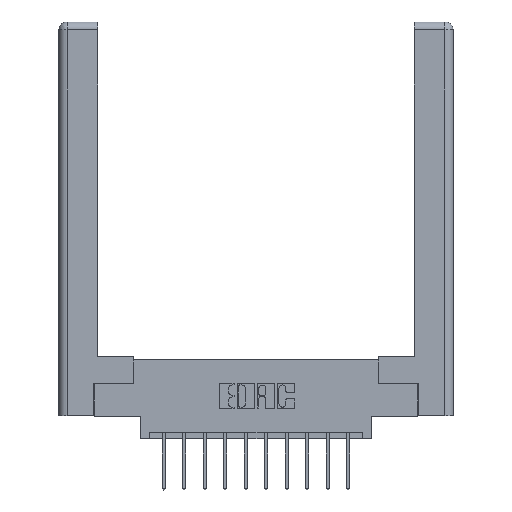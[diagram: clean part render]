
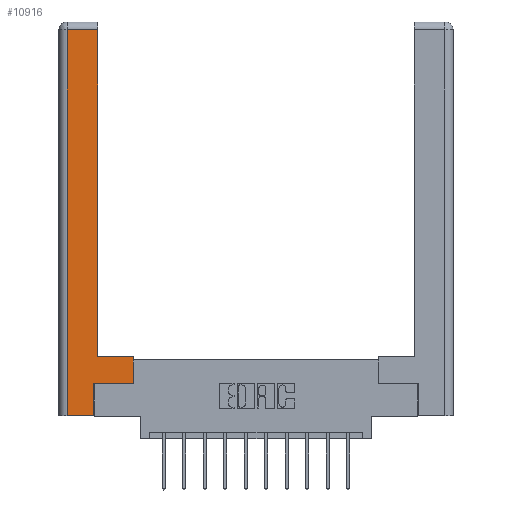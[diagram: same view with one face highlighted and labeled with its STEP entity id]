
A CAD part, top view. The second image highlights one B-rep face of the part: STEP entity #10916.
In plain terms, the highlighted planar face has unit normal (0, 0, 1).
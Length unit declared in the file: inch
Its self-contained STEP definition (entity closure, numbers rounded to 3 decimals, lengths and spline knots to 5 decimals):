
#333 = VECTOR ( 'NONE', #755, 39.37008 ) ;
#377 = LINE ( 'NONE', #9315, #12081 ) ;
#511 = VERTEX_POINT ( 'NONE', #4430 ) ;
#755 = DIRECTION ( 'NONE',  ( 0., -1., 0. ) ) ;
#834 = DIRECTION ( 'NONE',  ( -1., 0., 0. ) ) ;
#1196 = LINE ( 'NONE', #2316, #3840 ) ;
#1319 = VERTEX_POINT ( 'NONE', #8373 ) ;
#1495 = DIRECTION ( 'NONE',  ( -1., 0., 0. ) ) ;
#1690 = LINE ( 'NONE', #4418, #2929 ) ;
#2316 = CARTESIAN_POINT ( 'NONE',  ( 0.265, 0., 0. ) ) ;
#2762 = ORIENTED_EDGE ( 'NONE', *, *, #9810, .T. ) ;
#2822 = EDGE_CURVE ( 'NONE', #14529, #1319, #4258, .T. ) ;
#2929 = VECTOR ( 'NONE', #7453, 39.37008 ) ;
#3008 = FACE_OUTER_BOUND ( 'NONE', #6752, .T. ) ;
#3546 = EDGE_CURVE ( 'NONE', #511, #11935, #4234, .T. ) ;
#3840 = VECTOR ( 'NONE', #12680, 39.37008 ) ;
#3909 = PLANE ( 'NONE',  #6872 ) ;
#4000 = CARTESIAN_POINT ( 'NONE',  ( 0.295, 2.94, 0. ) ) ;
#4083 = CARTESIAN_POINT ( 'NONE',  ( 0.0615, 0., 0. ) ) ;
#4232 = ORIENTED_EDGE ( 'NONE', *, *, #2822, .T. ) ;
#4234 = LINE ( 'NONE', #9967, #333 ) ;
#4258 = LINE ( 'NONE', #5767, #7293 ) ;
#4418 = CARTESIAN_POINT ( 'NONE',  ( 0.265, 0.245, 0. ) ) ;
#4430 = CARTESIAN_POINT ( 'NONE',  ( 0.0615, 2.94, 0. ) ) ;
#4433 = CARTESIAN_POINT ( 'NONE',  ( 0.295, 0.45, 0. ) ) ;
#4456 = LINE ( 'NONE', #5331, #5339 ) ;
#4597 = CARTESIAN_POINT ( 'NONE',  ( 0.565, 0.45, 0. ) ) ;
#4698 = DIRECTION ( 'NONE',  ( 0., 1., 0. ) ) ;
#5149 = LINE ( 'NONE', #12906, #12946 ) ;
#5331 = CARTESIAN_POINT ( 'NONE',  ( 0.0615, 2.94, 0. ) ) ;
#5339 = VECTOR ( 'NONE', #834, 39.37008 ) ;
#5767 = CARTESIAN_POINT ( 'NONE',  ( 0.565, 0.245, 0. ) ) ;
#6020 = DIRECTION ( 'NONE',  ( -1., 0., 0. ) ) ;
#6538 = ORIENTED_EDGE ( 'NONE', *, *, #12284, .T. ) ;
#6570 = ORIENTED_EDGE ( 'NONE', *, *, #8959, .T. ) ;
#6721 = VERTEX_POINT ( 'NONE', #4597 ) ;
#6752 = EDGE_LOOP ( 'NONE', ( #6570, #8140, #14511, #6538, #13121, #4232, #2762, #13319 ) ) ;
#6872 = AXIS2_PLACEMENT_3D ( 'NONE', #14090, #10619, #1495 ) ;
#7293 = VECTOR ( 'NONE', #12496, 39.37008 ) ;
#7317 = DIRECTION ( 'NONE',  ( 0., 1., 0. ) ) ;
#7453 = DIRECTION ( 'NONE',  ( 0., 1., 0. ) ) ;
#8140 = ORIENTED_EDGE ( 'NONE', *, *, #9294, .T. ) ;
#8185 = VERTEX_POINT ( 'NONE', #4000 ) ;
#8361 = CARTESIAN_POINT ( 'NONE',  ( 0.295, 0.45, 0. ) ) ;
#8373 = CARTESIAN_POINT ( 'NONE',  ( 0.565, 0.245, 0. ) ) ;
#8959 = EDGE_CURVE ( 'NONE', #11451, #8185, #377, .T. ) ;
#9294 = EDGE_CURVE ( 'NONE', #8185, #511, #4456, .T. ) ;
#9315 = CARTESIAN_POINT ( 'NONE',  ( 0.295, 3., 0. ) ) ;
#9810 = EDGE_CURVE ( 'NONE', #1319, #6721, #5149, .T. ) ;
#9967 = CARTESIAN_POINT ( 'NONE',  ( 0.0615, 0., 0. ) ) ;
#10031 = VECTOR ( 'NONE', #6020, 39.37008 ) ;
#10619 = DIRECTION ( 'NONE',  ( 0., 0., -1. ) ) ;
#10916 = ADVANCED_FACE ( 'NONE', ( #3008 ), #3909, .F. ) ;
#11289 = CARTESIAN_POINT ( 'NONE',  ( 0.265, 0.245, 0. ) ) ;
#11451 = VERTEX_POINT ( 'NONE', #4433 ) ;
#11935 = VERTEX_POINT ( 'NONE', #4083 ) ;
#12081 = VECTOR ( 'NONE', #4698, 39.37008 ) ;
#12284 = EDGE_CURVE ( 'NONE', #11935, #14353, #1196, .T. ) ;
#12496 = DIRECTION ( 'NONE',  ( 1., 0., 0. ) ) ;
#12680 = DIRECTION ( 'NONE',  ( 1., 0., 0. ) ) ;
#12690 = LINE ( 'NONE', #8361, #10031 ) ;
#12906 = CARTESIAN_POINT ( 'NONE',  ( 0.565, 0.45, 0. ) ) ;
#12946 = VECTOR ( 'NONE', #7317, 39.37008 ) ;
#13115 = CARTESIAN_POINT ( 'NONE',  ( 0.265, 0., 0. ) ) ;
#13121 = ORIENTED_EDGE ( 'NONE', *, *, #14066, .T. ) ;
#13154 = EDGE_CURVE ( 'NONE', #6721, #11451, #12690, .T. ) ;
#13319 = ORIENTED_EDGE ( 'NONE', *, *, #13154, .T. ) ;
#14066 = EDGE_CURVE ( 'NONE', #14353, #14529, #1690, .T. ) ;
#14090 = CARTESIAN_POINT ( 'NONE',  ( 0., 0., 0. ) ) ;
#14353 = VERTEX_POINT ( 'NONE', #13115 ) ;
#14511 = ORIENTED_EDGE ( 'NONE', *, *, #3546, .T. ) ;
#14529 = VERTEX_POINT ( 'NONE', #11289 ) ;
